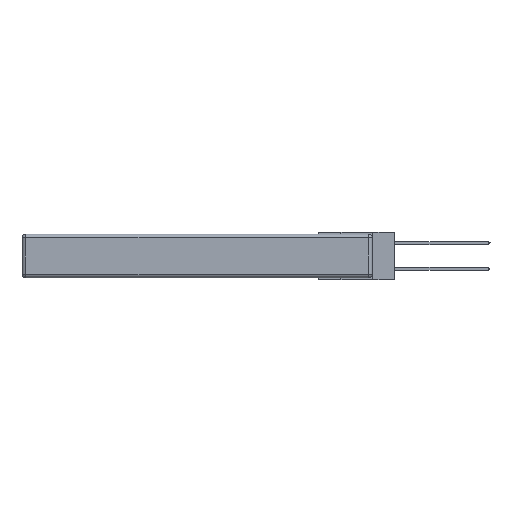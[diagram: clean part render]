
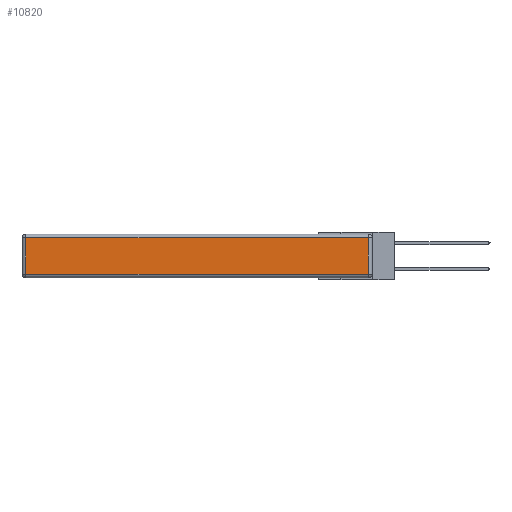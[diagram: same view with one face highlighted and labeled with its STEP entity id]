
A CAD part, left-side view. The second image highlights one B-rep face of the part: STEP entity #10820.
In plain terms, the highlighted planar face has unit normal (-1, 0, 0).
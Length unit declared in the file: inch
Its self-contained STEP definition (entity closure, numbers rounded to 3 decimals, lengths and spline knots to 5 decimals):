
#133 = CARTESIAN_POINT ( 'NONE',  ( 0., 2.72, -0.03 ) ) ;
#608 = CARTESIAN_POINT ( 'NONE',  ( 0., 2.72, -0.313 ) ) ;
#773 = CARTESIAN_POINT ( 'NONE',  ( 0., 0.03, -0.343 ) ) ;
#1683 = AXIS2_PLACEMENT_3D ( 'NONE', #7836, #4151, #6666 ) ;
#2071 = VERTEX_POINT ( 'NONE', #8701 ) ;
#2509 = VERTEX_POINT ( 'NONE', #133 ) ;
#3591 = ORIENTED_EDGE ( 'NONE', *, *, #15180, .T. ) ;
#3774 = EDGE_LOOP ( 'NONE', ( #4982, #3591, #5843, #12010 ) ) ;
#3818 = VERTEX_POINT ( 'NONE', #15952 ) ;
#4151 = DIRECTION ( 'NONE',  ( -1., 0., 0. ) ) ;
#4302 = VECTOR ( 'NONE', #14529, 39.37008 ) ;
#4522 = FACE_OUTER_BOUND ( 'NONE', #3774, .T. ) ;
#4982 = ORIENTED_EDGE ( 'NONE', *, *, #15578, .T. ) ;
#5649 = DIRECTION ( 'NONE',  ( 0., -1., 0. ) ) ;
#5843 = ORIENTED_EDGE ( 'NONE', *, *, #13347, .T. ) ;
#6666 = DIRECTION ( 'NONE',  ( 0., 0., 1. ) ) ;
#7125 = VECTOR ( 'NONE', #9304, 39.37008 ) ;
#7637 = LINE ( 'NONE', #773, #4302 ) ;
#7836 = CARTESIAN_POINT ( 'NONE',  ( 0., 0., -0.343 ) ) ;
#8701 = CARTESIAN_POINT ( 'NONE',  ( 0., 0.03, -0.03 ) ) ;
#8970 = PLANE ( 'NONE',  #1683 ) ;
#9304 = DIRECTION ( 'NONE',  ( 0., 1., 0. ) ) ;
#9358 = CARTESIAN_POINT ( 'NONE',  ( 0., 2.75, -0.03 ) ) ;
#10429 = LINE ( 'NONE', #9358, #7125 ) ;
#10569 = VECTOR ( 'NONE', #14449, 39.37008 ) ;
#10820 = ADVANCED_FACE ( 'NONE', ( #4522 ), #8970, .T. ) ;
#11988 = CARTESIAN_POINT ( 'NONE',  ( 0., 2.72, -0.343 ) ) ;
#12010 = ORIENTED_EDGE ( 'NONE', *, *, #15623, .T. ) ;
#12161 = LINE ( 'NONE', #11988, #10569 ) ;
#12848 = VECTOR ( 'NONE', #5649, 39.37008 ) ;
#13115 = CARTESIAN_POINT ( 'NONE',  ( 0., 0., -0.313 ) ) ;
#13347 = EDGE_CURVE ( 'NONE', #2071, #2509, #10429, .T. ) ;
#14449 = DIRECTION ( 'NONE',  ( 0., 0., -1. ) ) ;
#14529 = DIRECTION ( 'NONE',  ( 0., 0., 1. ) ) ;
#15180 = EDGE_CURVE ( 'NONE', #3818, #2071, #7637, .T. ) ;
#15496 = VERTEX_POINT ( 'NONE', #608 ) ;
#15578 = EDGE_CURVE ( 'NONE', #15496, #3818, #16086, .T. ) ;
#15623 = EDGE_CURVE ( 'NONE', #2509, #15496, #12161, .T. ) ;
#15952 = CARTESIAN_POINT ( 'NONE',  ( 0., 0.03, -0.313 ) ) ;
#16086 = LINE ( 'NONE', #13115, #12848 ) ;
